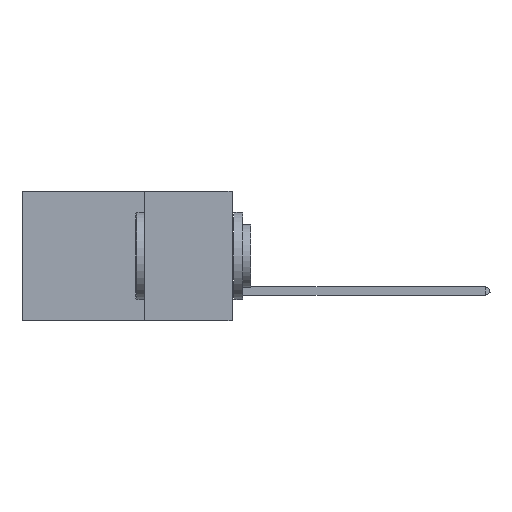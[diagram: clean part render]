
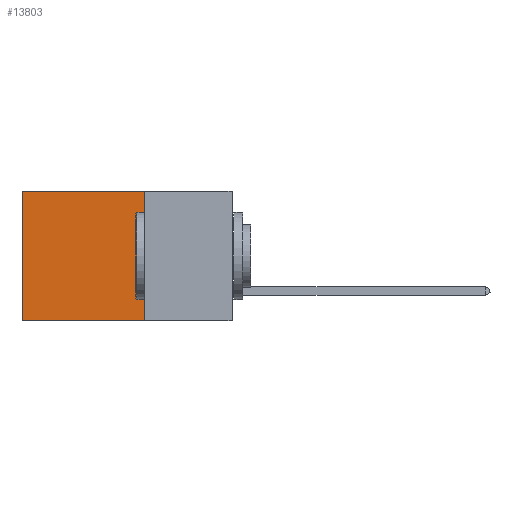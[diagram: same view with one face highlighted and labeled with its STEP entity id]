
A CAD part, left-side view. The second image highlights one B-rep face of the part: STEP entity #13803.
In plain terms, the highlighted planar face has unit normal (-1, 0, 0).
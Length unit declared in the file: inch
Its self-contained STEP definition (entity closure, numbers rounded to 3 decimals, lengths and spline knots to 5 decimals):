
#592 = VERTEX_POINT ( 'NONE', #3395 ) ;
#657 = ORIENTED_EDGE ( 'NONE', *, *, #4521, .T. ) ;
#880 = EDGE_CURVE ( 'NONE', #2272, #15601, #9658, .T. ) ;
#1097 = CARTESIAN_POINT ( 'NONE',  ( 0.2875, 0.25, 0. ) ) ;
#1496 = CARTESIAN_POINT ( 'NONE',  ( 0.2875, 0.6, 0. ) ) ;
#1573 = ORIENTED_EDGE ( 'NONE', *, *, #8930, .T. ) ;
#1620 = CARTESIAN_POINT ( 'NONE',  ( 0.2875, 0.25, 0. ) ) ;
#1662 = DIRECTION ( 'NONE',  ( 0., 0., -1. ) ) ;
#1730 = LINE ( 'NONE', #9217, #14233 ) ;
#1894 = CARTESIAN_POINT ( 'NONE',  ( 0.2875, 0.25, 0. ) ) ;
#2272 = VERTEX_POINT ( 'NONE', #13050 ) ;
#2301 = FACE_OUTER_BOUND ( 'NONE', #3236, .T. ) ;
#3220 = VECTOR ( 'NONE', #8045, 39.37008 ) ;
#3236 = EDGE_LOOP ( 'NONE', ( #1573, #8437, #9869, #657 ) ) ;
#3395 = CARTESIAN_POINT ( 'NONE',  ( 0.2875, 0.6, -0.37 ) ) ;
#4521 = EDGE_CURVE ( 'NONE', #2272, #9047, #5382, .T. ) ;
#5382 = LINE ( 'NONE', #1620, #3220 ) ;
#6271 = CARTESIAN_POINT ( 'NONE',  ( 0.2875, 0.25, -0.37 ) ) ;
#7714 = AXIS2_PLACEMENT_3D ( 'NONE', #1894, #7732, #15089 ) ;
#7725 = VECTOR ( 'NONE', #14755, 39.37008 ) ;
#7732 = DIRECTION ( 'NONE',  ( 1., 0., 0. ) ) ;
#8045 = DIRECTION ( 'NONE',  ( 0., 1., 0. ) ) ;
#8365 = DIRECTION ( 'NONE',  ( 0., 1., 0. ) ) ;
#8437 = ORIENTED_EDGE ( 'NONE', *, *, #14579, .F. ) ;
#8930 = EDGE_CURVE ( 'NONE', #9047, #592, #1730, .T. ) ;
#9047 = VERTEX_POINT ( 'NONE', #1496 ) ;
#9217 = CARTESIAN_POINT ( 'NONE',  ( 0.2875, 0.6, 0. ) ) ;
#9658 = LINE ( 'NONE', #1097, #7725 ) ;
#9869 = ORIENTED_EDGE ( 'NONE', *, *, #880, .F. ) ;
#12257 = VECTOR ( 'NONE', #8365, 39.37008 ) ;
#13050 = CARTESIAN_POINT ( 'NONE',  ( 0.2875, 0.25, 0. ) ) ;
#13376 = CARTESIAN_POINT ( 'NONE',  ( 0.2875, 0.25, -0.37 ) ) ;
#13803 = ADVANCED_FACE ( 'NONE', ( #2301 ), #14516, .F. ) ;
#14233 = VECTOR ( 'NONE', #1662, 39.37008 ) ;
#14516 = PLANE ( 'NONE',  #7714 ) ;
#14579 = EDGE_CURVE ( 'NONE', #15601, #592, #14599, .T. ) ;
#14599 = LINE ( 'NONE', #13376, #12257 ) ;
#14755 = DIRECTION ( 'NONE',  ( 0., 0., -1. ) ) ;
#15089 = DIRECTION ( 'NONE',  ( 0., 0., -1. ) ) ;
#15601 = VERTEX_POINT ( 'NONE', #6271 ) ;
